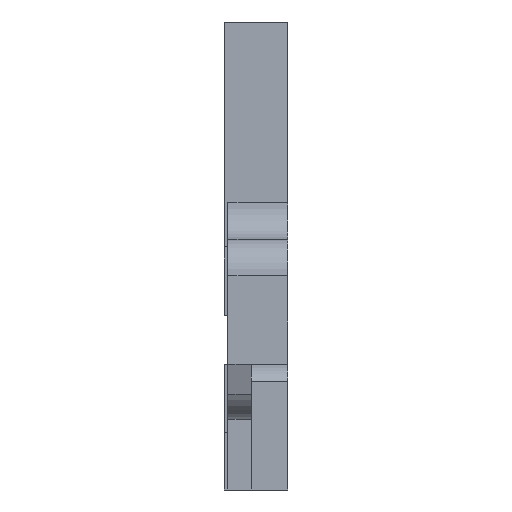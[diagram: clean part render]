
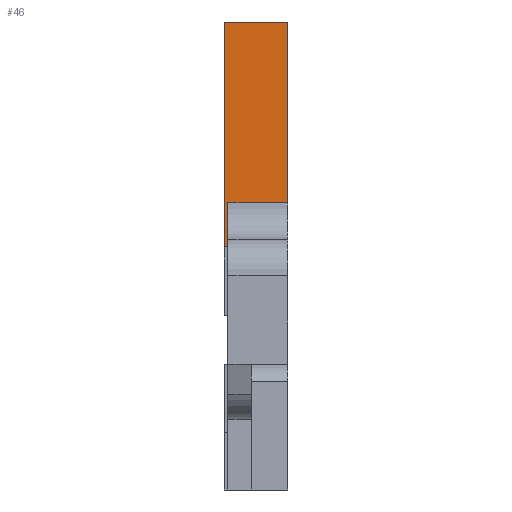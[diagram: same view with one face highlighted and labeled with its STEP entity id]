
A CAD part, left-side view. The second image highlights one B-rep face of the part: STEP entity #46.
In plain terms, the highlighted planar face has unit normal (-1, 0, 0).
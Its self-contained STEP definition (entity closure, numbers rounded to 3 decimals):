
#46 = ADVANCED_FACE ( 'NONE', ( #566 ), #250, .T. ) ;
#47 = VERTEX_POINT ( 'NONE', #2115 ) ;
#71 = DIRECTION ( 'NONE',  ( 0., 0., 1. ) ) ;
#250 = PLANE ( 'NONE',  #2835 ) ;
#302 = CARTESIAN_POINT ( 'NONE',  ( -1.5, -8.783, -24.88 ) ) ;
#355 = CARTESIAN_POINT ( 'NONE',  ( -1.5, -0.029, 0. ) ) ;
#492 = VECTOR ( 'NONE', #3154, 1000. ) ;
#530 = VERTEX_POINT ( 'NONE', #1907 ) ;
#566 = FACE_OUTER_BOUND ( 'NONE', #3094, .T. ) ;
#610 = VERTEX_POINT ( 'NONE', #3613 ) ;
#643 = LINE ( 'NONE', #2346, #1899 ) ;
#742 = EDGE_CURVE ( 'NONE', #47, #610, #2164, .T. ) ;
#797 = DIRECTION ( 'NONE',  ( 0., 0., 1. ) ) ;
#844 = CARTESIAN_POINT ( 'NONE',  ( -1.5, 30.937, -30.931 ) ) ;
#990 = LINE ( 'NONE', #2669, #3437 ) ;
#1216 = EDGE_CURVE ( 'NONE', #610, #530, #1331, .T. ) ;
#1281 = DIRECTION ( 'NONE',  ( 0., -1., 0. ) ) ;
#1331 = LINE ( 'NONE', #2581, #2707 ) ;
#1440 = ORIENTED_EDGE ( 'NONE', *, *, #742, .T. ) ;
#1469 = DIRECTION ( 'NONE',  ( 0., -1., 0. ) ) ;
#1534 = EDGE_CURVE ( 'NONE', #530, #2616, #3588, .T. ) ;
#1605 = DIRECTION ( 'NONE',  ( 0., 0., 1. ) ) ;
#1838 = LINE ( 'NONE', #1855, #492 ) ;
#1855 = CARTESIAN_POINT ( 'NONE',  ( -1.5, 29.762, 0. ) ) ;
#1899 = VECTOR ( 'NONE', #71, 1000. ) ;
#1907 = CARTESIAN_POINT ( 'NONE',  ( -1.5, -0.533, -24.88 ) ) ;
#2115 = CARTESIAN_POINT ( 'NONE',  ( -1.5, -0.029, -30.931 ) ) ;
#2164 = LINE ( 'NONE', #844, #3120 ) ;
#2167 = ORIENTED_EDGE ( 'NONE', *, *, #3263, .F. ) ;
#2239 = ORIENTED_EDGE ( 'NONE', *, *, #1216, .T. ) ;
#2287 = ORIENTED_EDGE ( 'NONE', *, *, #3885, .F. ) ;
#2303 = VECTOR ( 'NONE', #1281, 1000. ) ;
#2346 = CARTESIAN_POINT ( 'NONE',  ( -1.5, -0.029, -24.88 ) ) ;
#2379 = VERTEX_POINT ( 'NONE', #355 ) ;
#2496 = VERTEX_POINT ( 'NONE', #3765 ) ;
#2519 = ORIENTED_EDGE ( 'NONE', *, *, #1534, .T. ) ;
#2581 = CARTESIAN_POINT ( 'NONE',  ( -1.5, -0.533, -24.88 ) ) ;
#2616 = VERTEX_POINT ( 'NONE', #3906 ) ;
#2669 = CARTESIAN_POINT ( 'NONE',  ( -1.5, -8.783, 0. ) ) ;
#2707 = VECTOR ( 'NONE', #1605, 1000. ) ;
#2740 = EDGE_CURVE ( 'NONE', #47, #2379, #643, .T. ) ;
#2802 = CARTESIAN_POINT ( 'NONE',  ( -1.5, 29.762, 0. ) ) ;
#2835 = AXIS2_PLACEMENT_3D ( 'NONE', #2802, #3748, #797 ) ;
#3055 = DIRECTION ( 'NONE',  ( 0., 0., -1. ) ) ;
#3094 = EDGE_LOOP ( 'NONE', ( #2239, #2519, #2287, #2167, #3752, #1440 ) ) ;
#3120 = VECTOR ( 'NONE', #1469, 1000. ) ;
#3154 = DIRECTION ( 'NONE',  ( 0., -1., 0. ) ) ;
#3263 = EDGE_CURVE ( 'NONE', #2379, #2496, #1838, .T. ) ;
#3437 = VECTOR ( 'NONE', #3055, 1000. ) ;
#3588 = LINE ( 'NONE', #302, #2303 ) ;
#3613 = CARTESIAN_POINT ( 'NONE',  ( -1.5, -0.533, -30.931 ) ) ;
#3748 = DIRECTION ( 'NONE',  ( -1., 0., 0. ) ) ;
#3752 = ORIENTED_EDGE ( 'NONE', *, *, #2740, .F. ) ;
#3765 = CARTESIAN_POINT ( 'NONE',  ( -1.5, -8.783, 0. ) ) ;
#3885 = EDGE_CURVE ( 'NONE', #2496, #2616, #990, .T. ) ;
#3906 = CARTESIAN_POINT ( 'NONE',  ( -1.5, -8.783, -24.88 ) ) ;
